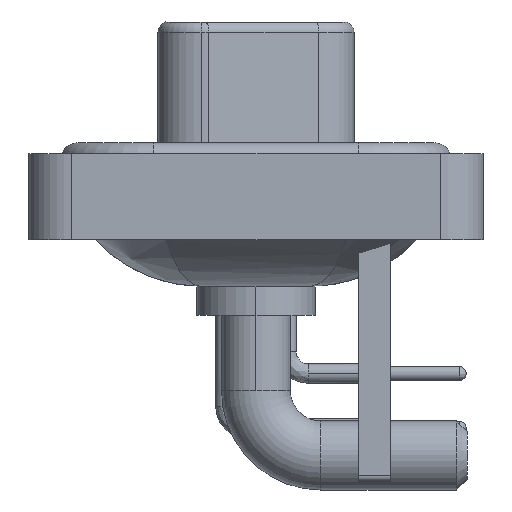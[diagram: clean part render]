
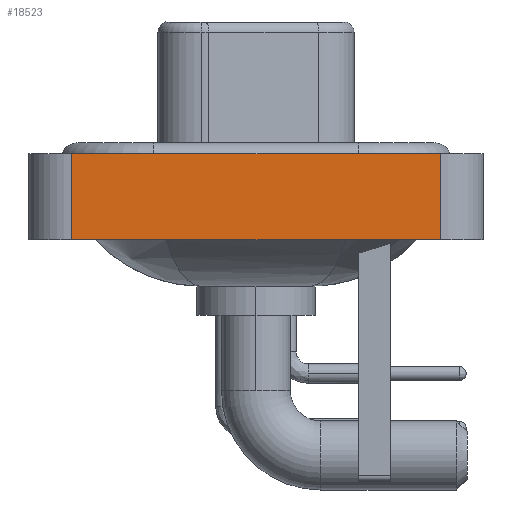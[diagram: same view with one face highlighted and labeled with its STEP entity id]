
A CAD part, left-side view. The second image highlights one B-rep face of the part: STEP entity #18523.
In plain terms, the highlighted planar face has unit normal (-1, 0, 0).
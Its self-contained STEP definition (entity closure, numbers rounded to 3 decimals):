
#307 = CARTESIAN_POINT ( 'NONE',  ( -7.3, -8.55, 0.4 ) ) ;
#2538 = VERTEX_POINT ( 'NONE', #18315 ) ;
#3219 = FACE_OUTER_BOUND ( 'NONE', #24965, .T. ) ;
#4155 = ORIENTED_EDGE ( 'NONE', *, *, #25054, .T. ) ;
#4295 = VECTOR ( 'NONE', #22919, 1000. ) ;
#4346 = ORIENTED_EDGE ( 'NONE', *, *, #16309, .F. ) ;
#4727 = ORIENTED_EDGE ( 'NONE', *, *, #13632, .T. ) ;
#6110 = PLANE ( 'NONE',  #10767 ) ;
#6171 = DIRECTION ( 'NONE',  ( 0., -1., 0. ) ) ;
#7832 = CARTESIAN_POINT ( 'NONE',  ( -7.3, 8.55, 0.4 ) ) ;
#8336 = VERTEX_POINT ( 'NONE', #13642 ) ;
#9085 = CARTESIAN_POINT ( 'NONE',  ( -7.3, -8.55, -3.6 ) ) ;
#10448 = DIRECTION ( 'NONE',  ( 0., 0., 1. ) ) ;
#10545 = VECTOR ( 'NONE', #6171, 1000. ) ;
#10767 = AXIS2_PLACEMENT_3D ( 'NONE', #9085, #16877, #14944 ) ;
#11444 = VERTEX_POINT ( 'NONE', #7832 ) ;
#11979 = LINE ( 'NONE', #20166, #13552 ) ;
#13143 = VERTEX_POINT ( 'NONE', #17925 ) ;
#13552 = VECTOR ( 'NONE', #10448, 1000. ) ;
#13632 = EDGE_CURVE ( 'NONE', #2538, #8336, #11979, .T. ) ;
#13642 = CARTESIAN_POINT ( 'NONE',  ( -7.3, -8.55, 0.4 ) ) ;
#13689 = LINE ( 'NONE', #307, #10545 ) ;
#14944 = DIRECTION ( 'NONE',  ( 0., 0., 1. ) ) ;
#15080 = CARTESIAN_POINT ( 'NONE',  ( -7.3, -8.55, -3.6 ) ) ;
#16309 = EDGE_CURVE ( 'NONE', #11444, #8336, #13689, .T. ) ;
#16460 = CARTESIAN_POINT ( 'NONE',  ( -7.3, 8.55, -3.6 ) ) ;
#16877 = DIRECTION ( 'NONE',  ( -1., 0., 0. ) ) ;
#17421 = VECTOR ( 'NONE', #18400, 1000. ) ;
#17925 = CARTESIAN_POINT ( 'NONE',  ( -7.3, 8.55, -3.6 ) ) ;
#18153 = ORIENTED_EDGE ( 'NONE', *, *, #23042, .F. ) ;
#18315 = CARTESIAN_POINT ( 'NONE',  ( -7.3, -8.55, -3.6 ) ) ;
#18400 = DIRECTION ( 'NONE',  ( 0., 0., 1. ) ) ;
#18523 = ADVANCED_FACE ( 'NONE', ( #3219 ), #6110, .T. ) ;
#20166 = CARTESIAN_POINT ( 'NONE',  ( -7.3, -8.55, -3.6 ) ) ;
#20309 = LINE ( 'NONE', #16460, #17421 ) ;
#22919 = DIRECTION ( 'NONE',  ( 0., -1., 0. ) ) ;
#23042 = EDGE_CURVE ( 'NONE', #13143, #11444, #20309, .T. ) ;
#24843 = LINE ( 'NONE', #15080, #4295 ) ;
#24965 = EDGE_LOOP ( 'NONE', ( #4727, #4346, #18153, #4155 ) ) ;
#25054 = EDGE_CURVE ( 'NONE', #13143, #2538, #24843, .T. ) ;
